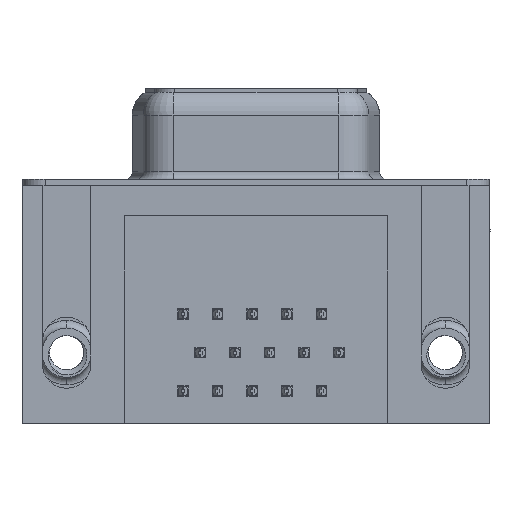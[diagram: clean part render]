
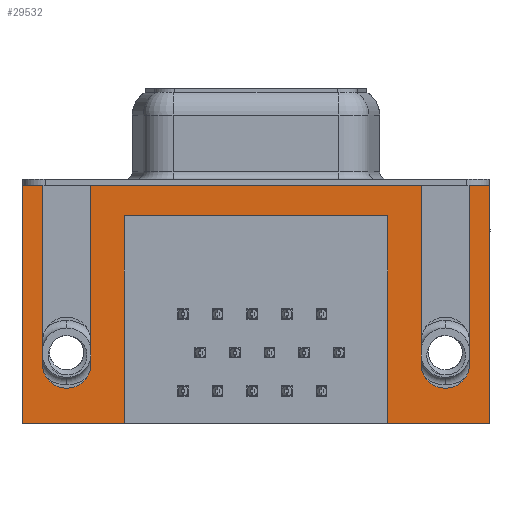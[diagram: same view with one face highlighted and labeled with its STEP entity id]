
A CAD part, front view. The second image highlights one B-rep face of the part: STEP entity #29532.
In plain terms, the highlighted planar face has unit normal (0, -1, 0).
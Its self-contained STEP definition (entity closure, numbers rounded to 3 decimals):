
#107 = DIRECTION ( 'NONE',  ( 0., 0., -1. ) ) ;
#493 = VECTOR ( 'NONE', #27952, 1000. ) ;
#1620 = AXIS2_PLACEMENT_3D ( 'NONE', #22420, #4387, #25469 ) ;
#2291 = VERTEX_POINT ( 'NONE', #30463 ) ;
#2786 = ORIENTED_EDGE ( 'NONE', *, *, #11983, .F. ) ;
#3076 = CARTESIAN_POINT ( 'NONE',  ( 21.2, -6.275, -2. ) ) ;
#3225 = VERTEX_POINT ( 'NONE', #20193 ) ;
#3298 = LINE ( 'NONE', #37216, #25434 ) ;
#3480 = ORIENTED_EDGE ( 'NONE', *, *, #20614, .F. ) ;
#3486 = EDGE_CURVE ( 'NONE', #12097, #24494, #34513, .T. ) ;
#3979 = CARTESIAN_POINT ( 'NONE',  ( 3.79, -6.275, -15.7 ) ) ;
#4189 = ORIENTED_EDGE ( 'NONE', *, *, #27032, .F. ) ;
#4325 = ORIENTED_EDGE ( 'NONE', *, *, #34944, .F. ) ;
#4387 = DIRECTION ( 'NONE',  ( 0., -1., 0. ) ) ;
#4573 = EDGE_CURVE ( 'NONE', #9043, #15333, #9802, .T. ) ;
#4617 = VECTOR ( 'NONE', #35704, 1000. ) ;
#5490 = CARTESIAN_POINT ( 'NONE',  ( 1.6, -6.275, 0. ) ) ;
#6029 = CARTESIAN_POINT ( 'NONE',  ( 3.79, -6.275, -2. ) ) ;
#6093 = VECTOR ( 'NONE', #26895, 1000. ) ;
#6756 = DIRECTION ( 'NONE',  ( 0., 0., 1. ) ) ;
#7121 = VERTEX_POINT ( 'NONE', #3979 ) ;
#7587 = LINE ( 'NONE', #34175, #23621 ) ;
#8079 = EDGE_CURVE ( 'NONE', #15333, #30213, #25633, .T. ) ;
#8482 = DIRECTION ( 'NONE',  ( 0., 0., 1. ) ) ;
#8885 = VECTOR ( 'NONE', #6756, 1000. ) ;
#9043 = VERTEX_POINT ( 'NONE', #33981 ) ;
#9679 = VERTEX_POINT ( 'NONE', #25677 ) ;
#9802 = LINE ( 'NONE', #18719, #8885 ) ;
#9806 = VERTEX_POINT ( 'NONE', #35375 ) ;
#10214 = DIRECTION ( 'NONE',  ( 0., 0., 1. ) ) ;
#10385 = CARTESIAN_POINT ( 'NONE',  ( 27.9, -6.275, -15.7 ) ) ;
#11450 = VERTEX_POINT ( 'NONE', #3076 ) ;
#11715 = CARTESIAN_POINT ( 'NONE',  ( 23.39, -6.275, 0. ) ) ;
#11983 = EDGE_CURVE ( 'NONE', #7121, #24922, #21686, .T. ) ;
#12000 = DIRECTION ( 'NONE',  ( 0., 0., -1. ) ) ;
#12097 = VERTEX_POINT ( 'NONE', #10385 ) ;
#12495 = VECTOR ( 'NONE', #17081, 1000. ) ;
#12626 = LINE ( 'NONE', #34585, #35863 ) ;
#12841 = CARTESIAN_POINT ( 'NONE',  ( -1.6, -6.275, -11.78 ) ) ;
#12972 = EDGE_CURVE ( 'NONE', #9806, #17330, #36357, .T. ) ;
#13295 = CARTESIAN_POINT ( 'NONE',  ( 24.99, -6.275, -11.78 ) ) ;
#13568 = CARTESIAN_POINT ( 'NONE',  ( 0., -6.275, -11.78 ) ) ;
#13901 = ORIENTED_EDGE ( 'NONE', *, *, #26777, .T. ) ;
#14016 = LINE ( 'NONE', #33184, #38187 ) ;
#14489 = ORIENTED_EDGE ( 'NONE', *, *, #26057, .F. ) ;
#14499 = DIRECTION ( 'NONE',  ( 1., 0., 0. ) ) ;
#14935 = LINE ( 'NONE', #15531, #31053 ) ;
#15333 = VERTEX_POINT ( 'NONE', #34124 ) ;
#15532 = ORIENTED_EDGE ( 'NONE', *, *, #3486, .F. ) ;
#15531 = CARTESIAN_POINT ( 'NONE',  ( 3.79, -6.275, -2. ) ) ;
#15544 = ORIENTED_EDGE ( 'NONE', *, *, #36870, .F. ) ;
#16035 = ORIENTED_EDGE ( 'NONE', *, *, #38420, .F. ) ;
#16305 = DIRECTION ( 'NONE',  ( -1., 0., 0. ) ) ;
#16468 = EDGE_CURVE ( 'NONE', #3225, #25733, #7587, .T. ) ;
#16586 = DIRECTION ( 'NONE',  ( 1., 0., 0. ) ) ;
#17081 = DIRECTION ( 'NONE',  ( 0., 0., 1. ) ) ;
#17220 = EDGE_CURVE ( 'NONE', #38556, #9679, #37805, .T. ) ;
#17330 = VERTEX_POINT ( 'NONE', #20045 ) ;
#18138 = ORIENTED_EDGE ( 'NONE', *, *, #12972, .F. ) ;
#18543 = CARTESIAN_POINT ( 'NONE',  ( 27.9, -6.275, -15.7 ) ) ;
#18585 = ORIENTED_EDGE ( 'NONE', *, *, #8079, .F. ) ;
#18719 = CARTESIAN_POINT ( 'NONE',  ( 26.59, -6.275, 0. ) ) ;
#19395 = PLANE ( 'NONE',  #1620 ) ;
#19526 = FACE_OUTER_BOUND ( 'NONE', #36209, .T. ) ;
#20045 = CARTESIAN_POINT ( 'NONE',  ( 23.39, -6.275, -11.78 ) ) ;
#20193 = CARTESIAN_POINT ( 'NONE',  ( -2.91, -6.275, 0. ) ) ;
#20541 = LINE ( 'NONE', #32224, #12495 ) ;
#20614 = EDGE_CURVE ( 'NONE', #24922, #3225, #20541, .T. ) ;
#20970 = ORIENTED_EDGE ( 'NONE', *, *, #16468, .F. ) ;
#21686 = LINE ( 'NONE', #18543, #493 ) ;
#22420 = CARTESIAN_POINT ( 'NONE',  ( -2.91, -6.275, -2.5 ) ) ;
#23621 = VECTOR ( 'NONE', #37206, 1000. ) ;
#23737 = VECTOR ( 'NONE', #14499, 1000. ) ;
#24066 = ORIENTED_EDGE ( 'NONE', *, *, #17220, .F. ) ;
#24494 = VERTEX_POINT ( 'NONE', #29633 ) ;
#24869 = ORIENTED_EDGE ( 'NONE', *, *, #25315, .F. ) ;
#24922 = VERTEX_POINT ( 'NONE', #30545 ) ;
#25315 = EDGE_CURVE ( 'NONE', #25733, #38556, #14016, .T. ) ;
#25434 = VECTOR ( 'NONE', #10214, 1000. ) ;
#25469 = DIRECTION ( 'NONE',  ( 0., 0., -1. ) ) ;
#25582 = CARTESIAN_POINT ( 'NONE',  ( 27.9, -6.275, -15.7 ) ) ;
#25633 = LINE ( 'NONE', #26423, #23737 ) ;
#25677 = CARTESIAN_POINT ( 'NONE',  ( 1.6, -6.275, -11.78 ) ) ;
#25733 = VERTEX_POINT ( 'NONE', #35399 ) ;
#26057 = EDGE_CURVE ( 'NONE', #26286, #9806, #12626, .T. ) ;
#26286 = VERTEX_POINT ( 'NONE', #5490 ) ;
#26423 = CARTESIAN_POINT ( 'NONE',  ( -2.91, -6.275, 0. ) ) ;
#26644 = AXIS2_PLACEMENT_3D ( 'NONE', #13568, #34764, #16586 ) ;
#26777 = EDGE_CURVE ( 'NONE', #12097, #30213, #28691, .T. ) ;
#26895 = DIRECTION ( 'NONE',  ( 0., 0., -1. ) ) ;
#27032 = EDGE_CURVE ( 'NONE', #11450, #2291, #14935, .T. ) ;
#27952 = DIRECTION ( 'NONE',  ( -1., 0., 0. ) ) ;
#28117 = CIRCLE ( 'NONE', #33005, 1.6 ) ;
#28390 = EDGE_CURVE ( 'NONE', #17330, #9043, #28117, .T. ) ;
#28691 = LINE ( 'NONE', #32674, #4617 ) ;
#29237 = VECTOR ( 'NONE', #107, 1000. ) ;
#29532 = ADVANCED_FACE ( 'NONE', ( #19526 ), #19395, .T. ) ;
#29609 = CARTESIAN_POINT ( 'NONE',  ( 21.2, -6.275, -2. ) ) ;
#29633 = CARTESIAN_POINT ( 'NONE',  ( 21.2, -6.275, -15.7 ) ) ;
#29851 = LINE ( 'NONE', #29609, #30789 ) ;
#30213 = VERTEX_POINT ( 'NONE', #38550 ) ;
#30463 = CARTESIAN_POINT ( 'NONE',  ( 3.79, -6.275, -2. ) ) ;
#30545 = CARTESIAN_POINT ( 'NONE',  ( -2.91, -6.275, -15.7 ) ) ;
#30789 = VECTOR ( 'NONE', #8482, 1000. ) ;
#31053 = VECTOR ( 'NONE', #36726, 1000. ) ;
#32160 = VECTOR ( 'NONE', #37643, 1000. ) ;
#32224 = CARTESIAN_POINT ( 'NONE',  ( -2.91, -6.275, -2.5 ) ) ;
#32674 = CARTESIAN_POINT ( 'NONE',  ( 27.9, -6.275, -2.5 ) ) ;
#33005 = AXIS2_PLACEMENT_3D ( 'NONE', #13295, #34489, #16305 ) ;
#33184 = CARTESIAN_POINT ( 'NONE',  ( -1.6, -6.275, 0. ) ) ;
#33981 = CARTESIAN_POINT ( 'NONE',  ( 26.59, -6.275, -11.78 ) ) ;
#34124 = CARTESIAN_POINT ( 'NONE',  ( 26.59, -6.275, 0. ) ) ;
#34175 = CARTESIAN_POINT ( 'NONE',  ( -2.91, -6.275, 0. ) ) ;
#34287 = ORIENTED_EDGE ( 'NONE', *, *, #4573, .F. ) ;
#34489 = DIRECTION ( 'NONE',  ( 0., -1., 0. ) ) ;
#34513 = LINE ( 'NONE', #25582, #32160 ) ;
#34585 = CARTESIAN_POINT ( 'NONE',  ( -2.91, -6.275, 0. ) ) ;
#34764 = DIRECTION ( 'NONE',  ( 0., -1., 0. ) ) ;
#34944 = EDGE_CURVE ( 'NONE', #24494, #11450, #29851, .T. ) ;
#35375 = CARTESIAN_POINT ( 'NONE',  ( 23.39, -6.275, 0. ) ) ;
#35399 = CARTESIAN_POINT ( 'NONE',  ( -1.6, -6.275, 0. ) ) ;
#35704 = DIRECTION ( 'NONE',  ( 0., 0., 1. ) ) ;
#35863 = VECTOR ( 'NONE', #37605, 1000. ) ;
#36209 = EDGE_LOOP ( 'NONE', ( #34287, #36659, #18138, #14489, #15544, #24066, #24869, #20970, #3480, #2786, #16035, #4189, #4325, #15532, #13901, #18585 ) ) ;
#36357 = LINE ( 'NONE', #11715, #6093 ) ;
#36659 = ORIENTED_EDGE ( 'NONE', *, *, #28390, .F. ) ;
#36726 = DIRECTION ( 'NONE',  ( -1., 0., 0. ) ) ;
#36870 = EDGE_CURVE ( 'NONE', #9679, #26286, #3298, .T. ) ;
#37206 = DIRECTION ( 'NONE',  ( 1., 0., 0. ) ) ;
#37216 = CARTESIAN_POINT ( 'NONE',  ( 1.6, -6.275, 0. ) ) ;
#37300 = LINE ( 'NONE', #6029, #29237 ) ;
#37605 = DIRECTION ( 'NONE',  ( 1., 0., 0. ) ) ;
#37643 = DIRECTION ( 'NONE',  ( -1., 0., 0. ) ) ;
#37805 = CIRCLE ( 'NONE', #26644, 1.6 ) ;
#38187 = VECTOR ( 'NONE', #12000, 1000. ) ;
#38420 = EDGE_CURVE ( 'NONE', #2291, #7121, #37300, .T. ) ;
#38550 = CARTESIAN_POINT ( 'NONE',  ( 27.9, -6.275, 0. ) ) ;
#38556 = VERTEX_POINT ( 'NONE', #12841 ) ;
